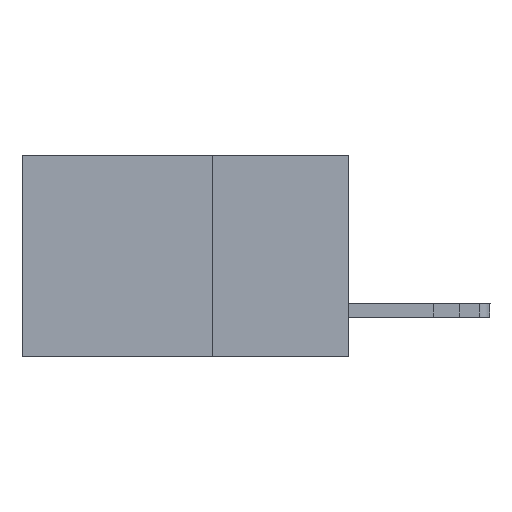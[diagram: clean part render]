
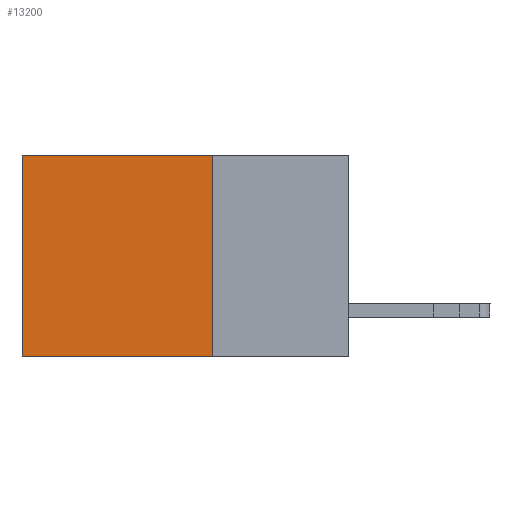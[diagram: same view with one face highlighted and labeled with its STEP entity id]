
A CAD part, left-side view. The second image highlights one B-rep face of the part: STEP entity #13200.
In plain terms, the highlighted planar face has unit normal (-1, 0, 0).
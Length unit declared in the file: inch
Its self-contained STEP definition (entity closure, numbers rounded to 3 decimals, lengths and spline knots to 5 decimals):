
#207 = LINE ( 'NONE', #13063, #15482 ) ;
#542 = ORIENTED_EDGE ( 'NONE', *, *, #754, .F. ) ;
#754 = EDGE_CURVE ( 'NONE', #10513, #9221, #207, .T. ) ;
#801 = LINE ( 'NONE', #11042, #6957 ) ;
#1606 = DIRECTION ( 'NONE',  ( 0., 1., 0. ) ) ;
#2013 = CARTESIAN_POINT ( 'NONE',  ( 0.298, 0.25, 0. ) ) ;
#2530 = ORIENTED_EDGE ( 'NONE', *, *, #7643, .T. ) ;
#4321 = VERTEX_POINT ( 'NONE', #14990 ) ;
#4371 = DIRECTION ( 'NONE',  ( 0., 0., -1. ) ) ;
#6156 = VECTOR ( 'NONE', #4371, 39.37008 ) ;
#6184 = PLANE ( 'NONE',  #13845 ) ;
#6957 = VECTOR ( 'NONE', #9647, 39.37008 ) ;
#7028 = VERTEX_POINT ( 'NONE', #13426 ) ;
#7124 = CARTESIAN_POINT ( 'NONE',  ( 0.298, 0.25, -0.37 ) ) ;
#7582 = VECTOR ( 'NONE', #12226, 39.37008 ) ;
#7643 = EDGE_CURVE ( 'NONE', #4321, #7028, #11764, .T. ) ;
#9167 = EDGE_CURVE ( 'NONE', #7028, #9221, #11113, .T. ) ;
#9221 = VERTEX_POINT ( 'NONE', #11099 ) ;
#9601 = ORIENTED_EDGE ( 'NONE', *, *, #9167, .T. ) ;
#9647 = DIRECTION ( 'NONE',  ( 0., 0., -1. ) ) ;
#10513 = VERTEX_POINT ( 'NONE', #7124 ) ;
#11042 = CARTESIAN_POINT ( 'NONE',  ( 0.298, 0.25, 0. ) ) ;
#11099 = CARTESIAN_POINT ( 'NONE',  ( 0.298, 0.6, -0.37 ) ) ;
#11113 = LINE ( 'NONE', #15749, #6156 ) ;
#11764 = LINE ( 'NONE', #2013, #7582 ) ;
#12226 = DIRECTION ( 'NONE',  ( 0., 1., 0. ) ) ;
#12307 = FACE_OUTER_BOUND ( 'NONE', #13688, .T. ) ;
#12536 = DIRECTION ( 'NONE',  ( 1., 0., 0. ) ) ;
#13063 = CARTESIAN_POINT ( 'NONE',  ( 0.298, 0.25, -0.37 ) ) ;
#13065 = EDGE_CURVE ( 'NONE', #4321, #10513, #801, .T. ) ;
#13200 = ADVANCED_FACE ( 'NONE', ( #12307 ), #6184, .F. ) ;
#13426 = CARTESIAN_POINT ( 'NONE',  ( 0.298, 0.6, 0. ) ) ;
#13688 = EDGE_LOOP ( 'NONE', ( #9601, #542, #15567, #2530 ) ) ;
#13845 = AXIS2_PLACEMENT_3D ( 'NONE', #15056, #12536, #16310 ) ;
#14990 = CARTESIAN_POINT ( 'NONE',  ( 0.298, 0.25, 0. ) ) ;
#15056 = CARTESIAN_POINT ( 'NONE',  ( 0.298, 0.25, 0. ) ) ;
#15482 = VECTOR ( 'NONE', #1606, 39.37008 ) ;
#15567 = ORIENTED_EDGE ( 'NONE', *, *, #13065, .F. ) ;
#15749 = CARTESIAN_POINT ( 'NONE',  ( 0.298, 0.6, 0. ) ) ;
#16310 = DIRECTION ( 'NONE',  ( 0., 0., -1. ) ) ;
